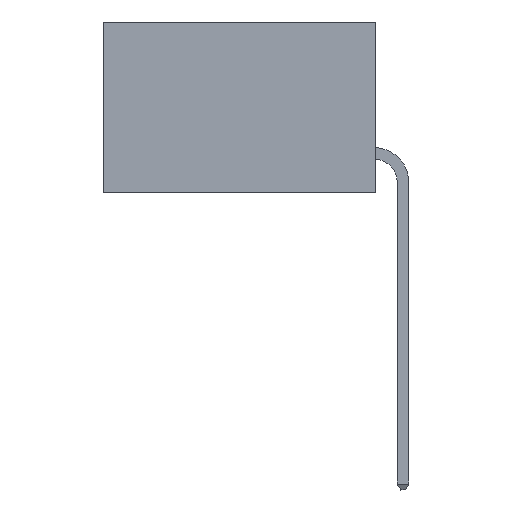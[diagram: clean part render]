
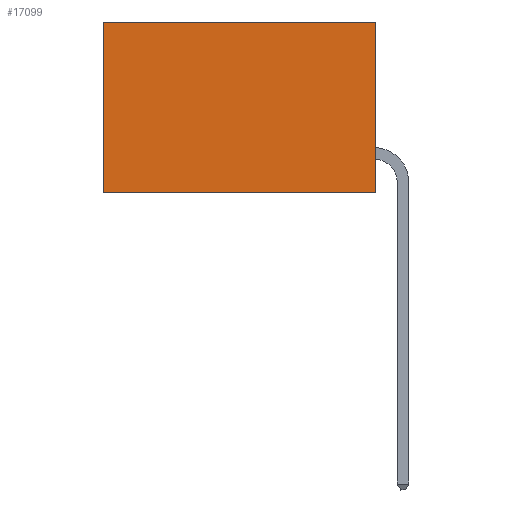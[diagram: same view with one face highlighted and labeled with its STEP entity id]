
A CAD part, left-side view. The second image highlights one B-rep face of the part: STEP entity #17099.
In plain terms, the highlighted planar face has unit normal (-1, 0, 0).
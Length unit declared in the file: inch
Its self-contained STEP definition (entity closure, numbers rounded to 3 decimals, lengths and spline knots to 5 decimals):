
#362 = CARTESIAN_POINT ( 'NONE',  ( 0.277, 0., -0.37 ) ) ;
#367 = VERTEX_POINT ( 'NONE', #15234 ) ;
#530 = VECTOR ( 'NONE', #14530, 39.37008 ) ;
#1096 = LINE ( 'NONE', #15066, #5212 ) ;
#2075 = DIRECTION ( 'NONE',  ( 1., 0., 0. ) ) ;
#2963 = CARTESIAN_POINT ( 'NONE',  ( 0.277, 0.59, -0.37 ) ) ;
#3643 = DIRECTION ( 'NONE',  ( 0., 0., -1. ) ) ;
#3694 = CARTESIAN_POINT ( 'NONE',  ( 0.277, 0.59, -0.37 ) ) ;
#3826 = EDGE_CURVE ( 'NONE', #21773, #5832, #9855, .T. ) ;
#4496 = ORIENTED_EDGE ( 'NONE', *, *, #10464, .T. ) ;
#4537 = DIRECTION ( 'NONE',  ( 0., 1., 0. ) ) ;
#5212 = VECTOR ( 'NONE', #6382, 39.37008 ) ;
#5832 = VERTEX_POINT ( 'NONE', #20626 ) ;
#6382 = DIRECTION ( 'NONE',  ( 0., 0., -1. ) ) ;
#8993 = LINE ( 'NONE', #3694, #22184 ) ;
#9193 = ORIENTED_EDGE ( 'NONE', *, *, #15681, .F. ) ;
#9855 = LINE ( 'NONE', #16676, #530 ) ;
#10464 = EDGE_CURVE ( 'NONE', #5832, #13768, #8993, .T. ) ;
#12258 = LINE ( 'NONE', #13296, #16813 ) ;
#12601 = AXIS2_PLACEMENT_3D ( 'NONE', #362, #2075, #14356 ) ;
#13296 = CARTESIAN_POINT ( 'NONE',  ( 0.277, 0., -0.37 ) ) ;
#13488 = EDGE_CURVE ( 'NONE', #21773, #367, #1096, .T. ) ;
#13768 = VERTEX_POINT ( 'NONE', #2963 ) ;
#13841 = FACE_OUTER_BOUND ( 'NONE', #20805, .T. ) ;
#14356 = DIRECTION ( 'NONE',  ( 0., 0., -1. ) ) ;
#14363 = ORIENTED_EDGE ( 'NONE', *, *, #3826, .T. ) ;
#14530 = DIRECTION ( 'NONE',  ( 0., 1., 0. ) ) ;
#15066 = CARTESIAN_POINT ( 'NONE',  ( 0.277, 0., -0.37 ) ) ;
#15234 = CARTESIAN_POINT ( 'NONE',  ( 0.277, 0., -0.37 ) ) ;
#15681 = EDGE_CURVE ( 'NONE', #367, #13768, #12258, .T. ) ;
#16676 = CARTESIAN_POINT ( 'NONE',  ( 0.277, 0., 0. ) ) ;
#16813 = VECTOR ( 'NONE', #4537, 39.37008 ) ;
#17099 = ADVANCED_FACE ( 'NONE', ( #13841 ), #21161, .F. ) ;
#18371 = ORIENTED_EDGE ( 'NONE', *, *, #13488, .F. ) ;
#20626 = CARTESIAN_POINT ( 'NONE',  ( 0.277, 0.59, 0. ) ) ;
#20805 = EDGE_LOOP ( 'NONE', ( #4496, #9193, #18371, #14363 ) ) ;
#21161 = PLANE ( 'NONE',  #12601 ) ;
#21748 = CARTESIAN_POINT ( 'NONE',  ( 0.277, 0., 0. ) ) ;
#21773 = VERTEX_POINT ( 'NONE', #21748 ) ;
#22184 = VECTOR ( 'NONE', #3643, 39.37008 ) ;
